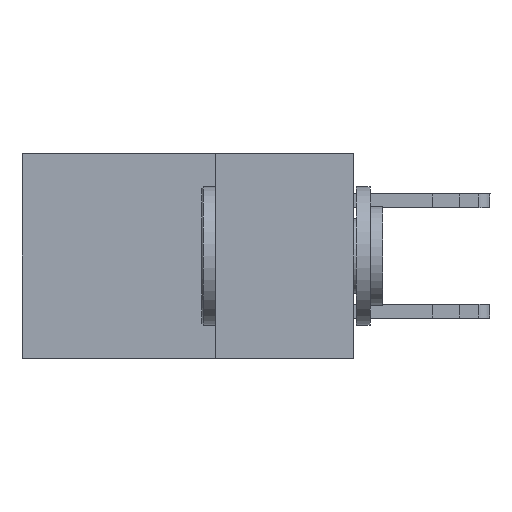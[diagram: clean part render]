
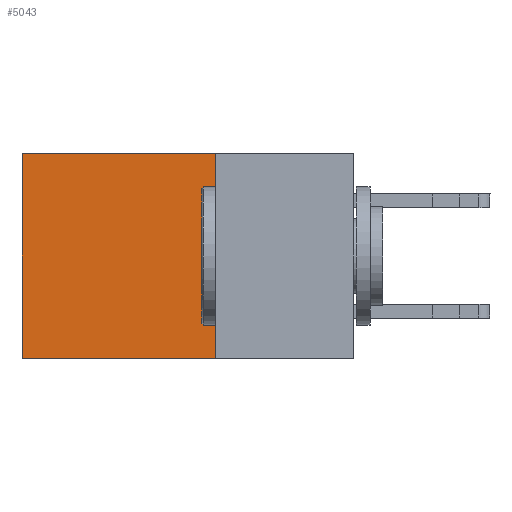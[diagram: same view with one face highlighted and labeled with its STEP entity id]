
A CAD part, left-side view. The second image highlights one B-rep face of the part: STEP entity #5043.
In plain terms, the highlighted planar face has unit normal (-1, 0, 0).
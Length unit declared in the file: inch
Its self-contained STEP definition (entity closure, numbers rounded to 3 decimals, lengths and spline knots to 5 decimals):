
#874 = EDGE_CURVE ( 'NONE', #14675, #5379, #26284, .T. ) ;
#927 = PLANE ( 'NONE',  #9859 ) ;
#930 = LINE ( 'NONE', #6578, #16313 ) ;
#3258 = DIRECTION ( 'NONE',  ( 1., 0., 0. ) ) ;
#3481 = DIRECTION ( 'NONE',  ( 0., 0., -1. ) ) ;
#4229 = ORIENTED_EDGE ( 'NONE', *, *, #26781, .T. ) ;
#5043 = ADVANCED_FACE ( 'NONE', ( #8478 ), #927, .F. ) ;
#5379 = VERTEX_POINT ( 'NONE', #10254 ) ;
#6578 = CARTESIAN_POINT ( 'NONE',  ( 0.2875, 0.25, -0.37 ) ) ;
#7799 = EDGE_CURVE ( 'NONE', #10771, #13826, #23384, .T. ) ;
#8426 = DIRECTION ( 'NONE',  ( 0., 0., -1. ) ) ;
#8478 = FACE_OUTER_BOUND ( 'NONE', #10494, .T. ) ;
#8546 = CARTESIAN_POINT ( 'NONE',  ( 0.2875, 0.6, 0. ) ) ;
#9859 = AXIS2_PLACEMENT_3D ( 'NONE', #25112, #3258, #8426 ) ;
#10254 = CARTESIAN_POINT ( 'NONE',  ( 0.2875, 0.6, -0.37 ) ) ;
#10494 = EDGE_LOOP ( 'NONE', ( #16147, #25457, #16176, #4229 ) ) ;
#10771 = VERTEX_POINT ( 'NONE', #17068 ) ;
#13826 = VERTEX_POINT ( 'NONE', #31472 ) ;
#14223 = DIRECTION ( 'NONE',  ( 0., 1., 0. ) ) ;
#14675 = VERTEX_POINT ( 'NONE', #27889 ) ;
#15826 = VECTOR ( 'NONE', #22115, 39.37008 ) ;
#16147 = ORIENTED_EDGE ( 'NONE', *, *, #874, .T. ) ;
#16176 = ORIENTED_EDGE ( 'NONE', *, *, #7799, .F. ) ;
#16313 = VECTOR ( 'NONE', #14223, 39.37008 ) ;
#17068 = CARTESIAN_POINT ( 'NONE',  ( 0.2875, 0.25, 0. ) ) ;
#17886 = VECTOR ( 'NONE', #22076, 39.37008 ) ;
#18345 = EDGE_CURVE ( 'NONE', #13826, #5379, #930, .T. ) ;
#22069 = CARTESIAN_POINT ( 'NONE',  ( 0.2875, 0.25, 0. ) ) ;
#22076 = DIRECTION ( 'NONE',  ( 0., 1., 0. ) ) ;
#22115 = DIRECTION ( 'NONE',  ( 0., 0., -1. ) ) ;
#23384 = LINE ( 'NONE', #29645, #15826 ) ;
#24337 = LINE ( 'NONE', #22069, #17886 ) ;
#25112 = CARTESIAN_POINT ( 'NONE',  ( 0.2875, 0.25, 0. ) ) ;
#25457 = ORIENTED_EDGE ( 'NONE', *, *, #18345, .F. ) ;
#25903 = VECTOR ( 'NONE', #3481, 39.37008 ) ;
#26284 = LINE ( 'NONE', #8546, #25903 ) ;
#26781 = EDGE_CURVE ( 'NONE', #10771, #14675, #24337, .T. ) ;
#27889 = CARTESIAN_POINT ( 'NONE',  ( 0.2875, 0.6, 0. ) ) ;
#29645 = CARTESIAN_POINT ( 'NONE',  ( 0.2875, 0.25, 0. ) ) ;
#31472 = CARTESIAN_POINT ( 'NONE',  ( 0.2875, 0.25, -0.37 ) ) ;
